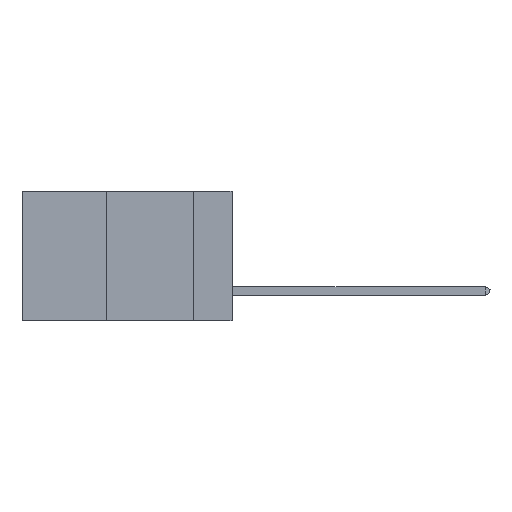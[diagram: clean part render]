
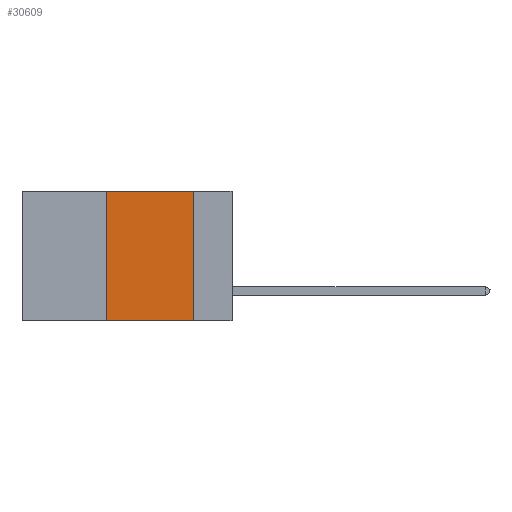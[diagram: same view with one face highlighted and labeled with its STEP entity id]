
A CAD part, left-side view. The second image highlights one B-rep face of the part: STEP entity #30609.
In plain terms, the highlighted planar face has unit normal (-1, 0, 0).
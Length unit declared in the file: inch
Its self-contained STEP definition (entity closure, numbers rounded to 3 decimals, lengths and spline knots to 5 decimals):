
#351 = CARTESIAN_POINT ( 'NONE',  ( 0., 0.11, -0.37 ) ) ;
#1786 = ORIENTED_EDGE ( 'NONE', *, *, #4828, .F. ) ;
#2703 = CARTESIAN_POINT ( 'NONE',  ( 0., 0.11, 0. ) ) ;
#4007 = CARTESIAN_POINT ( 'NONE',  ( 0., 0.36, -0.37 ) ) ;
#4566 = CARTESIAN_POINT ( 'NONE',  ( 0., 0.11, 0. ) ) ;
#4828 = EDGE_CURVE ( 'NONE', #34462, #15037, #11564, .T. ) ;
#6375 = EDGE_CURVE ( 'NONE', #34462, #36326, #6501, .T. ) ;
#6496 = FACE_OUTER_BOUND ( 'NONE', #12058, .T. ) ;
#6501 = LINE ( 'NONE', #21883, #41415 ) ;
#6550 = VECTOR ( 'NONE', #23756, 39.37008 ) ;
#8076 = CARTESIAN_POINT ( 'NONE',  ( 0., 0.6, 0. ) ) ;
#8886 = DIRECTION ( 'NONE',  ( 0., 0., 1. ) ) ;
#10160 = CARTESIAN_POINT ( 'NONE',  ( 0., 0.6, 0. ) ) ;
#11564 = LINE ( 'NONE', #12238, #33406 ) ;
#12055 = VERTEX_POINT ( 'NONE', #4566 ) ;
#12058 = EDGE_LOOP ( 'NONE', ( #44058, #26327, #1786, #33317 ) ) ;
#12238 = CARTESIAN_POINT ( 'NONE',  ( 0., 0.36, 0. ) ) ;
#15037 = VERTEX_POINT ( 'NONE', #32339 ) ;
#17050 = DIRECTION ( 'NONE',  ( 0., 0., -1. ) ) ;
#17355 = DIRECTION ( 'NONE',  ( 1., 0., 0. ) ) ;
#21883 = CARTESIAN_POINT ( 'NONE',  ( 0., 0.6, -0.37 ) ) ;
#23756 = DIRECTION ( 'NONE',  ( 0., 0., -1. ) ) ;
#25218 = EDGE_CURVE ( 'NONE', #15037, #12055, #39745, .T. ) ;
#26181 = LINE ( 'NONE', #2703, #6550 ) ;
#26327 = ORIENTED_EDGE ( 'NONE', *, *, #25218, .F. ) ;
#28813 = AXIS2_PLACEMENT_3D ( 'NONE', #10160, #17355, #17050 ) ;
#29182 = DIRECTION ( 'NONE',  ( 0., -1., 0. ) ) ;
#30609 = ADVANCED_FACE ( 'NONE', ( #6496 ), #41579, .F. ) ;
#32339 = CARTESIAN_POINT ( 'NONE',  ( 0., 0.36, 0. ) ) ;
#33317 = ORIENTED_EDGE ( 'NONE', *, *, #6375, .T. ) ;
#33406 = VECTOR ( 'NONE', #8886, 39.37008 ) ;
#34462 = VERTEX_POINT ( 'NONE', #4007 ) ;
#36326 = VERTEX_POINT ( 'NONE', #351 ) ;
#36737 = DIRECTION ( 'NONE',  ( 0., -1., 0. ) ) ;
#39745 = LINE ( 'NONE', #8076, #43025 ) ;
#41415 = VECTOR ( 'NONE', #29182, 39.37008 ) ;
#41579 = PLANE ( 'NONE',  #28813 ) ;
#43025 = VECTOR ( 'NONE', #36737, 39.37008 ) ;
#44058 = ORIENTED_EDGE ( 'NONE', *, *, #44485, .F. ) ;
#44485 = EDGE_CURVE ( 'NONE', #12055, #36326, #26181, .T. ) ;
